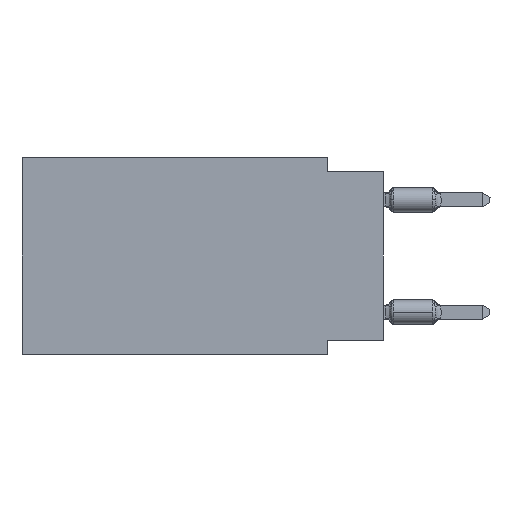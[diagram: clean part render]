
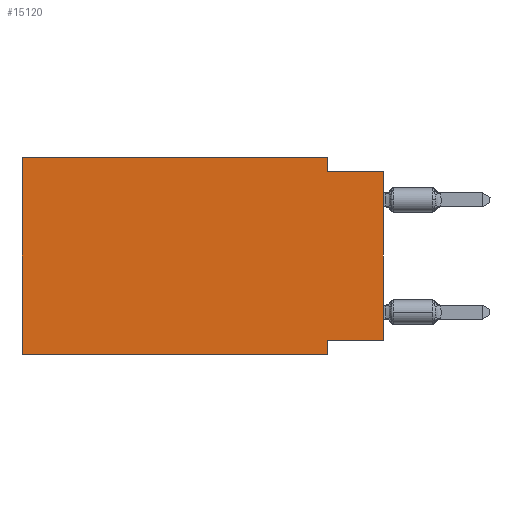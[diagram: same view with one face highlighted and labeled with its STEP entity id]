
A CAD part, left-side view. The second image highlights one B-rep face of the part: STEP entity #15120.
In plain terms, the highlighted planar face has unit normal (-1, 0, 0).
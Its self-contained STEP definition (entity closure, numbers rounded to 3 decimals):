
#594 = EDGE_CURVE ( 'NONE', #1805, #39021, #5788, .T. ) ;
#669 = VERTEX_POINT ( 'NONE', #27524 ) ;
#837 = VECTOR ( 'NONE', #39230, 1000. ) ;
#1766 = LINE ( 'NONE', #26701, #28498 ) ;
#1805 = VERTEX_POINT ( 'NONE', #32899 ) ;
#2626 = CARTESIAN_POINT ( 'NONE',  ( 0., 16.383, 0. ) ) ;
#2680 = VERTEX_POINT ( 'NONE', #28326 ) ;
#3400 = VERTEX_POINT ( 'NONE', #14776 ) ;
#3433 = VERTEX_POINT ( 'NONE', #5310 ) ;
#3537 = LINE ( 'NONE', #9986, #6012 ) ;
#4048 = EDGE_CURVE ( 'NONE', #28222, #669, #1766, .T. ) ;
#4407 = EDGE_CURVE ( 'NONE', #18082, #669, #3537, .T. ) ;
#4870 = ORIENTED_EDGE ( 'NONE', *, *, #18806, .F. ) ;
#5283 = CARTESIAN_POINT ( 'NONE',  ( 0., 16.383, 0. ) ) ;
#5310 = CARTESIAN_POINT ( 'NONE',  ( 0., 16.383, 0. ) ) ;
#5788 = LINE ( 'NONE', #29944, #8118 ) ;
#6012 = VECTOR ( 'NONE', #16209, 1000. ) ;
#7021 = DIRECTION ( 'NONE',  ( 0., 0., -1. ) ) ;
#7211 = DIRECTION ( 'NONE',  ( 1., 0., 0. ) ) ;
#7352 = LINE ( 'NONE', #19624, #35508 ) ;
#8118 = VECTOR ( 'NONE', #14667, 1000. ) ;
#9986 = CARTESIAN_POINT ( 'NONE',  ( 0., 16.383, -8.89 ) ) ;
#10488 = LINE ( 'NONE', #23134, #32314 ) ;
#11127 = DIRECTION ( 'NONE',  ( 0., -1., 0. ) ) ;
#11146 = EDGE_LOOP ( 'NONE', ( #30856, #38915, #13530, #13384, #39546, #26535, #14477, #4870 ) ) ;
#11212 = DIRECTION ( 'NONE',  ( 0., 0., -1. ) ) ;
#11774 = EDGE_CURVE ( 'NONE', #3433, #2680, #26613, .T. ) ;
#13384 = ORIENTED_EDGE ( 'NONE', *, *, #11774, .F. ) ;
#13530 = ORIENTED_EDGE ( 'NONE', *, *, #29677, .F. ) ;
#14477 = ORIENTED_EDGE ( 'NONE', *, *, #4048, .F. ) ;
#14667 = DIRECTION ( 'NONE',  ( 0., -1., 0. ) ) ;
#14776 = CARTESIAN_POINT ( 'NONE',  ( 0., 0., -8.255 ) ) ;
#15120 = ADVANCED_FACE ( 'NONE', ( #27944 ), #25320, .F. ) ;
#16209 = DIRECTION ( 'NONE',  ( 0., -1., 0. ) ) ;
#16446 = EDGE_CURVE ( 'NONE', #3400, #39021, #10488, .T. ) ;
#16725 = DIRECTION ( 'NONE',  ( 0., 0., 1. ) ) ;
#18082 = VERTEX_POINT ( 'NONE', #36028 ) ;
#18806 = EDGE_CURVE ( 'NONE', #3400, #28222, #7352, .T. ) ;
#19624 = CARTESIAN_POINT ( 'NONE',  ( 0., 0., -8.255 ) ) ;
#20544 = LINE ( 'NONE', #26184, #837 ) ;
#21914 = LINE ( 'NONE', #2626, #26017 ) ;
#23134 = CARTESIAN_POINT ( 'NONE',  ( 0., 0., 0. ) ) ;
#25320 = PLANE ( 'NONE',  #30030 ) ;
#26017 = VECTOR ( 'NONE', #36811, 1000. ) ;
#26184 = CARTESIAN_POINT ( 'NONE',  ( 0., 2.54, 0. ) ) ;
#26535 = ORIENTED_EDGE ( 'NONE', *, *, #4407, .T. ) ;
#26613 = LINE ( 'NONE', #5283, #33943 ) ;
#26701 = CARTESIAN_POINT ( 'NONE',  ( 0., 2.54, -8.89 ) ) ;
#27524 = CARTESIAN_POINT ( 'NONE',  ( 0., 2.54, -8.89 ) ) ;
#27944 = FACE_OUTER_BOUND ( 'NONE', #11146, .T. ) ;
#28222 = VERTEX_POINT ( 'NONE', #29836 ) ;
#28326 = CARTESIAN_POINT ( 'NONE',  ( 0., 2.54, 0. ) ) ;
#28498 = VECTOR ( 'NONE', #11212, 1000. ) ;
#29677 = EDGE_CURVE ( 'NONE', #2680, #1805, #20544, .T. ) ;
#29836 = CARTESIAN_POINT ( 'NONE',  ( 0., 2.54, -8.255 ) ) ;
#29944 = CARTESIAN_POINT ( 'NONE',  ( 0., 0., -0.635 ) ) ;
#30030 = AXIS2_PLACEMENT_3D ( 'NONE', #37186, #7211, #7021 ) ;
#30065 = DIRECTION ( 'NONE',  ( 0., 1., 0. ) ) ;
#30856 = ORIENTED_EDGE ( 'NONE', *, *, #16446, .T. ) ;
#32314 = VECTOR ( 'NONE', #16725, 1000. ) ;
#32371 = CARTESIAN_POINT ( 'NONE',  ( 0., 0., -0.635 ) ) ;
#32899 = CARTESIAN_POINT ( 'NONE',  ( 0., 2.54, -0.635 ) ) ;
#33943 = VECTOR ( 'NONE', #11127, 1000. ) ;
#35508 = VECTOR ( 'NONE', #30065, 1000. ) ;
#36028 = CARTESIAN_POINT ( 'NONE',  ( 0., 16.383, -8.89 ) ) ;
#36187 = EDGE_CURVE ( 'NONE', #18082, #3433, #21914, .T. ) ;
#36811 = DIRECTION ( 'NONE',  ( 0., 0., 1. ) ) ;
#37186 = CARTESIAN_POINT ( 'NONE',  ( 0., 16.383, 0. ) ) ;
#38915 = ORIENTED_EDGE ( 'NONE', *, *, #594, .F. ) ;
#39021 = VERTEX_POINT ( 'NONE', #32371 ) ;
#39230 = DIRECTION ( 'NONE',  ( 0., 0., -1. ) ) ;
#39546 = ORIENTED_EDGE ( 'NONE', *, *, #36187, .F. ) ;
